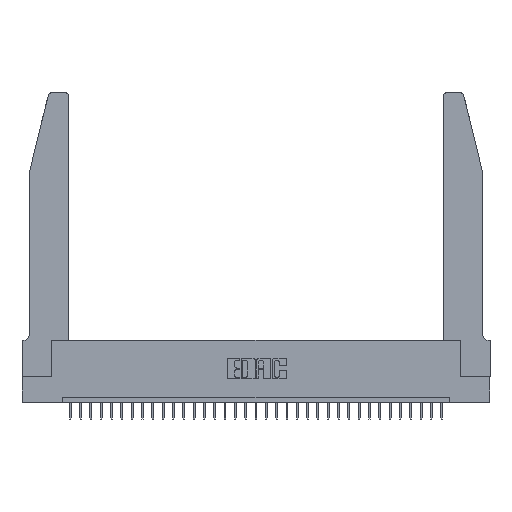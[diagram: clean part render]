
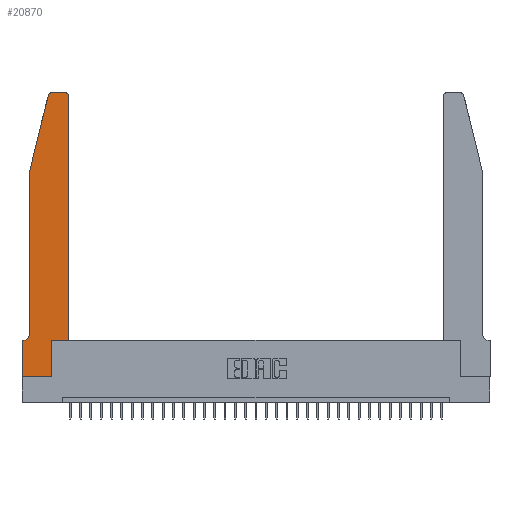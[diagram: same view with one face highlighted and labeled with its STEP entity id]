
A CAD part, top view. The second image highlights one B-rep face of the part: STEP entity #20870.
In plain terms, the highlighted planar face has unit normal (0, 0, 1).
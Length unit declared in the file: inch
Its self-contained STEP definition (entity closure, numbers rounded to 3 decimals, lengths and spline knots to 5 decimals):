
#755 = LINE ( 'NONE', #24631, #13196 ) ;
#789 = ORIENTED_EDGE ( 'NONE', *, *, #9228, .T. ) ;
#979 = DIRECTION ( 'NONE',  ( 0., 1., 0. ) ) ;
#1300 = VECTOR ( 'NONE', #11263, 39.37008 ) ;
#1614 = CIRCLE ( 'NONE', #5423, 0.07 ) ;
#1949 = DIRECTION ( 'NONE',  ( 1., 0., 0. ) ) ;
#3284 = VECTOR ( 'NONE', #14576, 39.37008 ) ;
#3395 = VERTEX_POINT ( 'NONE', #18883 ) ;
#3674 = LINE ( 'NONE', #27696, #13296 ) ;
#4327 = ORIENTED_EDGE ( 'NONE', *, *, #11613, .T. ) ;
#4795 = EDGE_CURVE ( 'NONE', #23350, #29340, #25308, .T. ) ;
#4919 = CIRCLE ( 'NONE', #10491, 0.03 ) ;
#4966 = DIRECTION ( 'NONE',  ( 1., 0., 0. ) ) ;
#5423 = AXIS2_PLACEMENT_3D ( 'NONE', #23591, #18293, #15817 ) ;
#5906 = CARTESIAN_POINT ( 'NONE',  ( 0.2865, 0., 0.37 ) ) ;
#6223 = VECTOR ( 'NONE', #22747, 39.37008 ) ;
#7085 = VERTEX_POINT ( 'NONE', #9836 ) ;
#7256 = DIRECTION ( 'NONE',  ( -0.239, -0.971, 0. ) ) ;
#7297 = EDGE_CURVE ( 'NONE', #11969, #32650, #17861, .T. ) ;
#7322 = AXIS2_PLACEMENT_3D ( 'NONE', #10125, #30612, #25419 ) ;
#7378 = LINE ( 'NONE', #9735, #13374 ) ;
#8204 = CARTESIAN_POINT ( 'NONE',  ( 0., 0.35, 0.37 ) ) ;
#8227 = CARTESIAN_POINT ( 'NONE',  ( 0.25487, 2.72718, 0.37 ) ) ;
#8846 = CARTESIAN_POINT ( 'NONE',  ( 0.4205, 2.75, 0.37 ) ) ;
#9228 = EDGE_CURVE ( 'NONE', #14085, #32675, #11873, .T. ) ;
#9585 = CARTESIAN_POINT ( 'NONE',  ( 0.4505, 2.72, 0.37 ) ) ;
#9735 = CARTESIAN_POINT ( 'NONE',  ( 0.0755, 2., 0.37 ) ) ;
#9836 = CARTESIAN_POINT ( 'NONE',  ( 0.2865, 0.35, 0.37 ) ) ;
#10099 = VECTOR ( 'NONE', #15479, 39.37008 ) ;
#10125 = CARTESIAN_POINT ( 'NONE',  ( 0.4205, 2.72, 0.37 ) ) ;
#10134 = DIRECTION ( 'NONE',  ( 0., 0., 1. ) ) ;
#10491 = AXIS2_PLACEMENT_3D ( 'NONE', #23139, #10134, #4966 ) ;
#11066 = CARTESIAN_POINT ( 'NONE',  ( 0.0055, 0.35, 0.37 ) ) ;
#11263 = DIRECTION ( 'NONE',  ( 1., 0., 0. ) ) ;
#11427 = CARTESIAN_POINT ( 'NONE',  ( 0.0755, 0.42, 0.37 ) ) ;
#11544 = CARTESIAN_POINT ( 'NONE',  ( 0.2605, 2.75, 0.37 ) ) ;
#11613 = EDGE_CURVE ( 'NONE', #32650, #3395, #25020, .T. ) ;
#11873 = LINE ( 'NONE', #20168, #6223 ) ;
#11969 = VERTEX_POINT ( 'NONE', #9585 ) ;
#11970 = EDGE_CURVE ( 'NONE', #28525, #31436, #3674, .T. ) ;
#12015 = EDGE_CURVE ( 'NONE', #21724, #11969, #16912, .T. ) ;
#12362 = CARTESIAN_POINT ( 'NONE',  ( 0.0755, 2., 0.37 ) ) ;
#12406 = AXIS2_PLACEMENT_3D ( 'NONE', #8204, #21142, #19352 ) ;
#12484 = ORIENTED_EDGE ( 'NONE', *, *, #4795, .T. ) ;
#13064 = ORIENTED_EDGE ( 'NONE', *, *, #28088, .T. ) ;
#13104 = EDGE_CURVE ( 'NONE', #32675, #28525, #755, .T. ) ;
#13196 = VECTOR ( 'NONE', #27247, 39.37008 ) ;
#13296 = VECTOR ( 'NONE', #1949, 39.37008 ) ;
#13374 = VECTOR ( 'NONE', #7256, 39.37008 ) ;
#13730 = PLANE ( 'NONE',  #12406 ) ;
#14085 = VERTEX_POINT ( 'NONE', #11066 ) ;
#14576 = DIRECTION ( 'NONE',  ( -1., 0., 0. ) ) ;
#14793 = FACE_OUTER_BOUND ( 'NONE', #26668, .T. ) ;
#14936 = DIRECTION ( 'NONE',  ( 0., -1., 0. ) ) ;
#15479 = DIRECTION ( 'NONE',  ( 0., 1., 0. ) ) ;
#15817 = DIRECTION ( 'NONE',  ( -1., 0., 0. ) ) ;
#16065 = ORIENTED_EDGE ( 'NONE', *, *, #24278, .T. ) ;
#16165 = CARTESIAN_POINT ( 'NONE',  ( 0., 0., 0.37 ) ) ;
#16405 = EDGE_CURVE ( 'NONE', #20700, #23350, #7378, .T. ) ;
#16425 = CARTESIAN_POINT ( 'NONE',  ( 0.2865, 0.35, 0.37 ) ) ;
#16845 = ORIENTED_EDGE ( 'NONE', *, *, #12015, .T. ) ;
#16912 = LINE ( 'NONE', #30294, #10099 ) ;
#17861 = CIRCLE ( 'NONE', #7322, 0.03 ) ;
#18077 = EDGE_CURVE ( 'NONE', #29340, #14085, #1614, .T. ) ;
#18293 = DIRECTION ( 'NONE',  ( 0., 0., -1. ) ) ;
#18721 = ORIENTED_EDGE ( 'NONE', *, *, #31935, .T. ) ;
#18883 = CARTESIAN_POINT ( 'NONE',  ( 0.284, 2.75, 0.37 ) ) ;
#18943 = CARTESIAN_POINT ( 'NONE',  ( 0., 0.35, 0.37 ) ) ;
#19352 = DIRECTION ( 'NONE',  ( 1., 0., 0. ) ) ;
#20168 = CARTESIAN_POINT ( 'NONE',  ( 0.0755, 0.35, 0.37 ) ) ;
#20557 = ORIENTED_EDGE ( 'NONE', *, *, #11970, .T. ) ;
#20700 = VERTEX_POINT ( 'NONE', #8227 ) ;
#20870 = ADVANCED_FACE ( 'NONE', ( #14793 ), #13730, .T. ) ;
#21142 = DIRECTION ( 'NONE',  ( 0., 0., 1. ) ) ;
#21724 = VERTEX_POINT ( 'NONE', #31353 ) ;
#22747 = DIRECTION ( 'NONE',  ( -1., 0., 0. ) ) ;
#23139 = CARTESIAN_POINT ( 'NONE',  ( 0.284, 2.72, 0.37 ) ) ;
#23350 = VERTEX_POINT ( 'NONE', #28135 ) ;
#23591 = CARTESIAN_POINT ( 'NONE',  ( 0.0055, 0.42, 0.37 ) ) ;
#23871 = ORIENTED_EDGE ( 'NONE', *, *, #7297, .T. ) ;
#24089 = CARTESIAN_POINT ( 'NONE',  ( 0.4505, 0.35, 0.37 ) ) ;
#24278 = EDGE_CURVE ( 'NONE', #3395, #20700, #4919, .T. ) ;
#24631 = CARTESIAN_POINT ( 'NONE',  ( 0., 0., 0.37 ) ) ;
#25020 = LINE ( 'NONE', #11544, #3284 ) ;
#25308 = LINE ( 'NONE', #12362, #30925 ) ;
#25419 = DIRECTION ( 'NONE',  ( 1., 0., 0. ) ) ;
#26211 = VECTOR ( 'NONE', #979, 39.37008 ) ;
#26438 = ORIENTED_EDGE ( 'NONE', *, *, #18077, .T. ) ;
#26668 = EDGE_LOOP ( 'NONE', ( #4327, #16065, #28005, #12484, #26438, #789, #28397, #20557, #13064, #18721, #16845, #23871 ) ) ;
#27247 = DIRECTION ( 'NONE',  ( 0., -1., 0. ) ) ;
#27696 = CARTESIAN_POINT ( 'NONE',  ( 0., 0., 0.37 ) ) ;
#28005 = ORIENTED_EDGE ( 'NONE', *, *, #16405, .T. ) ;
#28088 = EDGE_CURVE ( 'NONE', #31436, #7085, #33134, .T. ) ;
#28135 = CARTESIAN_POINT ( 'NONE',  ( 0.0755, 2., 0.37 ) ) ;
#28397 = ORIENTED_EDGE ( 'NONE', *, *, #13104, .T. ) ;
#28525 = VERTEX_POINT ( 'NONE', #16165 ) ;
#29340 = VERTEX_POINT ( 'NONE', #11427 ) ;
#30294 = CARTESIAN_POINT ( 'NONE',  ( 0.4505, 0.35, 0.37 ) ) ;
#30612 = DIRECTION ( 'NONE',  ( 0., 0., 1. ) ) ;
#30925 = VECTOR ( 'NONE', #14936, 39.37008 ) ;
#31063 = LINE ( 'NONE', #24089, #1300 ) ;
#31353 = CARTESIAN_POINT ( 'NONE',  ( 0.4505, 0.35, 0.37 ) ) ;
#31436 = VERTEX_POINT ( 'NONE', #5906 ) ;
#31935 = EDGE_CURVE ( 'NONE', #7085, #21724, #31063, .T. ) ;
#32650 = VERTEX_POINT ( 'NONE', #8846 ) ;
#32675 = VERTEX_POINT ( 'NONE', #18943 ) ;
#33134 = LINE ( 'NONE', #16425, #26211 ) ;
